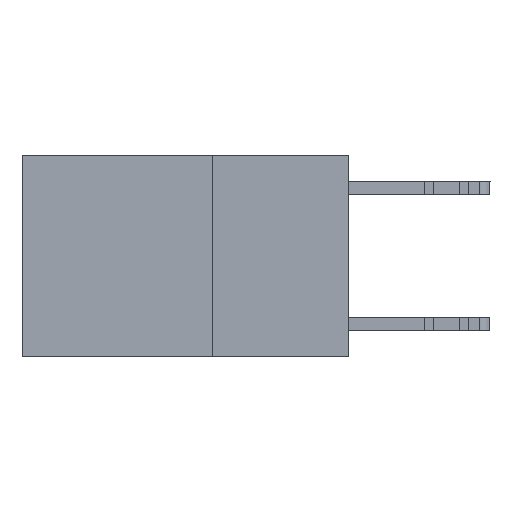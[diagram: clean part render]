
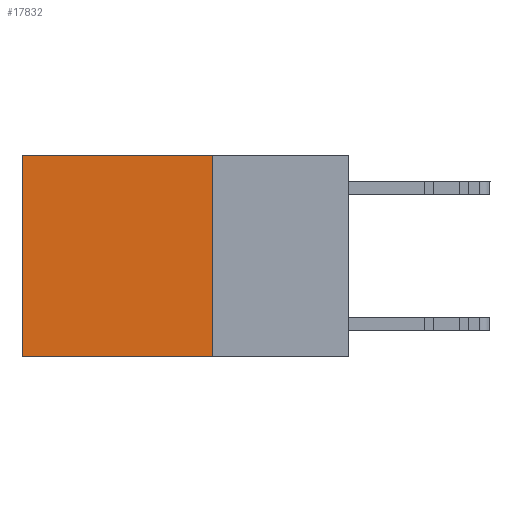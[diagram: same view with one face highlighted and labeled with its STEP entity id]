
A CAD part, left-side view. The second image highlights one B-rep face of the part: STEP entity #17832.
In plain terms, the highlighted planar face has unit normal (-1, 0, 0).
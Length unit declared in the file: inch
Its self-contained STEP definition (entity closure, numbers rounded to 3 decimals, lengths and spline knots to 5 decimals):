
#2337 = ORIENTED_EDGE ( 'NONE', *, *, #2772, .T. ) ;
#2772 = EDGE_CURVE ( 'NONE', #9838, #30599, #30092, .T. ) ;
#3090 = CARTESIAN_POINT ( 'NONE',  ( 0.2625, 0.6, 0. ) ) ;
#4868 = VERTEX_POINT ( 'NONE', #27094 ) ;
#5127 = CARTESIAN_POINT ( 'NONE',  ( 0.2625, 0.25, 0. ) ) ;
#6406 = CARTESIAN_POINT ( 'NONE',  ( 0.2625, 0.6, 0. ) ) ;
#7605 = DIRECTION ( 'NONE',  ( 1., 0., 0. ) ) ;
#7611 = DIRECTION ( 'NONE',  ( 0., 0., -1. ) ) ;
#8764 = CARTESIAN_POINT ( 'NONE',  ( 0.2625, 0.6, -0.37 ) ) ;
#9199 = ORIENTED_EDGE ( 'NONE', *, *, #26032, .F. ) ;
#9204 = AXIS2_PLACEMENT_3D ( 'NONE', #5127, #7605, #16884 ) ;
#9838 = VERTEX_POINT ( 'NONE', #23776 ) ;
#11072 = LINE ( 'NONE', #13089, #11375 ) ;
#11375 = VECTOR ( 'NONE', #22584, 39.37008 ) ;
#12697 = LINE ( 'NONE', #3090, #22163 ) ;
#13089 = CARTESIAN_POINT ( 'NONE',  ( 0.2625, 0.25, 0. ) ) ;
#15023 = EDGE_LOOP ( 'NONE', ( #17566, #15980, #9199, #2337 ) ) ;
#15962 = CARTESIAN_POINT ( 'NONE',  ( 0.2625, 0.25, 0. ) ) ;
#15980 = ORIENTED_EDGE ( 'NONE', *, *, #30410, .F. ) ;
#16611 = VERTEX_POINT ( 'NONE', #8764 ) ;
#16884 = DIRECTION ( 'NONE',  ( 0., 0., -1. ) ) ;
#17566 = ORIENTED_EDGE ( 'NONE', *, *, #19135, .T. ) ;
#17832 = ADVANCED_FACE ( 'NONE', ( #28696 ), #22041, .F. ) ;
#19135 = EDGE_CURVE ( 'NONE', #30599, #16611, #12697, .T. ) ;
#20065 = VECTOR ( 'NONE', #27917, 39.37008 ) ;
#20913 = CARTESIAN_POINT ( 'NONE',  ( 0.2625, 0.25, -0.37 ) ) ;
#22041 = PLANE ( 'NONE',  #9204 ) ;
#22163 = VECTOR ( 'NONE', #7611, 39.37008 ) ;
#22584 = DIRECTION ( 'NONE',  ( 0., 0., -1. ) ) ;
#23550 = LINE ( 'NONE', #20913, #27903 ) ;
#23776 = CARTESIAN_POINT ( 'NONE',  ( 0.2625, 0.25, 0. ) ) ;
#26032 = EDGE_CURVE ( 'NONE', #9838, #4868, #11072, .T. ) ;
#27094 = CARTESIAN_POINT ( 'NONE',  ( 0.2625, 0.25, -0.37 ) ) ;
#27903 = VECTOR ( 'NONE', #30353, 39.37008 ) ;
#27917 = DIRECTION ( 'NONE',  ( 0., 1., 0. ) ) ;
#28696 = FACE_OUTER_BOUND ( 'NONE', #15023, .T. ) ;
#30092 = LINE ( 'NONE', #15962, #20065 ) ;
#30353 = DIRECTION ( 'NONE',  ( 0., 1., 0. ) ) ;
#30410 = EDGE_CURVE ( 'NONE', #4868, #16611, #23550, .T. ) ;
#30599 = VERTEX_POINT ( 'NONE', #6406 ) ;
